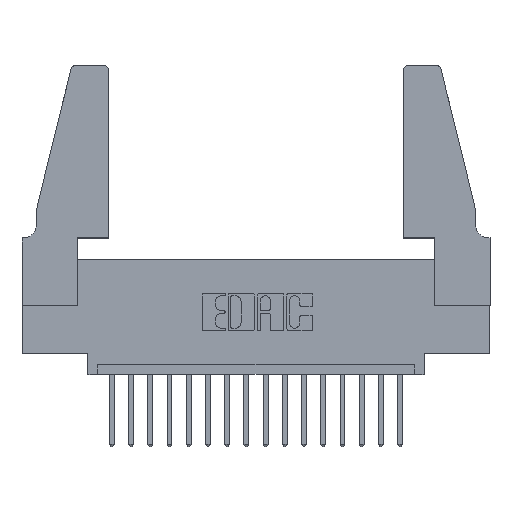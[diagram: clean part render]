
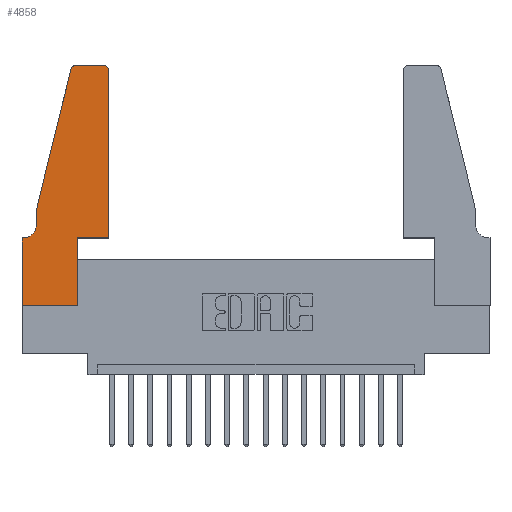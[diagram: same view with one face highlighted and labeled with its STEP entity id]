
A CAD part, top view. The second image highlights one B-rep face of the part: STEP entity #4858.
In plain terms, the highlighted planar face has unit normal (0, 0, 1).
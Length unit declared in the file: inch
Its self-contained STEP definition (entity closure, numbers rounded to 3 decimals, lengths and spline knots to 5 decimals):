
#25 = CARTESIAN_POINT ( 'NONE',  ( 0.4505, 0.35, 0.37 ) ) ;
#268 = EDGE_CURVE ( 'NONE', #8774, #3133, #7131, .T. ) ;
#560 = LINE ( 'NONE', #14806, #11050 ) ;
#875 = CARTESIAN_POINT ( 'NONE',  ( 0.2865, 0.35, 0.37 ) ) ;
#986 = CARTESIAN_POINT ( 'NONE',  ( 0.2865, 0.35, 0.37 ) ) ;
#1124 = EDGE_CURVE ( 'NONE', #5325, #8774, #1185, .T. ) ;
#1141 = ORIENTED_EDGE ( 'NONE', *, *, #7953, .T. ) ;
#1185 = LINE ( 'NONE', #986, #7198 ) ;
#1199 = DIRECTION ( 'NONE',  ( 1., 0., 0. ) ) ;
#1319 = VERTEX_POINT ( 'NONE', #6841 ) ;
#1401 = CARTESIAN_POINT ( 'NONE',  ( 0.0055, 0.42, 0.37 ) ) ;
#1741 = DIRECTION ( 'NONE',  ( -1., 0., 0. ) ) ;
#2296 = VECTOR ( 'NONE', #4685, 39.37008 ) ;
#2375 = DIRECTION ( 'NONE',  ( -1., 0., 0. ) ) ;
#2564 = ORIENTED_EDGE ( 'NONE', *, *, #8250, .T. ) ;
#2803 = DIRECTION ( 'NONE',  ( 1., 0., 0. ) ) ;
#3133 = VERTEX_POINT ( 'NONE', #7202 ) ;
#3313 = VECTOR ( 'NONE', #2375, 39.37008 ) ;
#3562 = VERTEX_POINT ( 'NONE', #12331 ) ;
#3579 = VERTEX_POINT ( 'NONE', #12566 ) ;
#3792 = CARTESIAN_POINT ( 'NONE',  ( 0., 0.35, 0.37 ) ) ;
#3866 = DIRECTION ( 'NONE',  ( 0., 1., 0. ) ) ;
#4262 = VERTEX_POINT ( 'NONE', #10989 ) ;
#4298 = CARTESIAN_POINT ( 'NONE',  ( 0.0755, 0.42, 0.37 ) ) ;
#4301 = AXIS2_PLACEMENT_3D ( 'NONE', #6587, #17739, #1199 ) ;
#4428 = LINE ( 'NONE', #6195, #2296 ) ;
#4685 = DIRECTION ( 'NONE',  ( -0.239, -0.971, 0. ) ) ;
#4858 = ADVANCED_FACE ( 'NONE', ( #16996 ), #9367, .T. ) ;
#4866 = LINE ( 'NONE', #14162, #9160 ) ;
#5049 = LINE ( 'NONE', #15166, #8493 ) ;
#5102 = CARTESIAN_POINT ( 'NONE',  ( 0.2865, 0., 0.37 ) ) ;
#5199 = CIRCLE ( 'NONE', #6097, 0.03 ) ;
#5325 = VERTEX_POINT ( 'NONE', #5102 ) ;
#5746 = DIRECTION ( 'NONE',  ( 1., 0., 0. ) ) ;
#6097 = AXIS2_PLACEMENT_3D ( 'NONE', #13949, #13835, #5746 ) ;
#6195 = CARTESIAN_POINT ( 'NONE',  ( 0.0755, 0.5, 0.37 ) ) ;
#6388 = DIRECTION ( 'NONE',  ( 0., 1., 0. ) ) ;
#6435 = ORIENTED_EDGE ( 'NONE', *, *, #17171, .T. ) ;
#6513 = ORIENTED_EDGE ( 'NONE', *, *, #9025, .T. ) ;
#6587 = CARTESIAN_POINT ( 'NONE',  ( 0.4205, 1.22, 0.37 ) ) ;
#6841 = CARTESIAN_POINT ( 'NONE',  ( 0., 0., 0.37 ) ) ;
#6978 = LINE ( 'NONE', #10558, #3313 ) ;
#7131 = LINE ( 'NONE', #25, #10958 ) ;
#7132 = DIRECTION ( 'NONE',  ( 0., -1., 0. ) ) ;
#7198 = VECTOR ( 'NONE', #6388, 39.37008 ) ;
#7202 = CARTESIAN_POINT ( 'NONE',  ( 0.4505, 0.35, 0.37 ) ) ;
#7537 = ORIENTED_EDGE ( 'NONE', *, *, #10752, .T. ) ;
#7682 = CARTESIAN_POINT ( 'NONE',  ( 0.0055, 0.35, 0.37 ) ) ;
#7765 = LINE ( 'NONE', #8574, #16847 ) ;
#7808 = EDGE_LOOP ( 'NONE', ( #1141, #11427, #2564, #12625, #10492, #16204, #7537, #12334, #12401, #11277, #6513, #6435 ) ) ;
#7953 = EDGE_CURVE ( 'NONE', #15549, #12107, #4866, .T. ) ;
#8250 = EDGE_CURVE ( 'NONE', #3579, #4262, #4428, .T. ) ;
#8289 = CARTESIAN_POINT ( 'NONE',  ( 0.4505, 1.22, 0.37 ) ) ;
#8493 = VECTOR ( 'NONE', #10809, 39.37008 ) ;
#8574 = CARTESIAN_POINT ( 'NONE',  ( 0., 0., 0.37 ) ) ;
#8774 = VERTEX_POINT ( 'NONE', #875 ) ;
#9025 = EDGE_CURVE ( 'NONE', #3133, #11017, #560, .T. ) ;
#9160 = VECTOR ( 'NONE', #1741, 39.37008 ) ;
#9367 = PLANE ( 'NONE',  #10485 ) ;
#9583 = EDGE_CURVE ( 'NONE', #11639, #3562, #6978, .T. ) ;
#10456 = EDGE_CURVE ( 'NONE', #12107, #3579, #5199, .T. ) ;
#10485 = AXIS2_PLACEMENT_3D ( 'NONE', #3792, #16322, #14791 ) ;
#10492 = ORIENTED_EDGE ( 'NONE', *, *, #13800, .T. ) ;
#10558 = CARTESIAN_POINT ( 'NONE',  ( 0.0755, 0.35, 0.37 ) ) ;
#10690 = CARTESIAN_POINT ( 'NONE',  ( 0.284, 1.25, 0.37 ) ) ;
#10752 = EDGE_CURVE ( 'NONE', #3562, #1319, #7765, .T. ) ;
#10809 = DIRECTION ( 'NONE',  ( 1., 0., 0. ) ) ;
#10958 = VECTOR ( 'NONE', #2803, 39.37008 ) ;
#10973 = DIRECTION ( 'NONE',  ( 0., 0., -1. ) ) ;
#10989 = CARTESIAN_POINT ( 'NONE',  ( 0.0755, 0.5, 0.37 ) ) ;
#11017 = VERTEX_POINT ( 'NONE', #8289 ) ;
#11050 = VECTOR ( 'NONE', #3866, 39.37008 ) ;
#11277 = ORIENTED_EDGE ( 'NONE', *, *, #268, .T. ) ;
#11427 = ORIENTED_EDGE ( 'NONE', *, *, #10456, .T. ) ;
#11463 = VERTEX_POINT ( 'NONE', #4298 ) ;
#11639 = VERTEX_POINT ( 'NONE', #7682 ) ;
#12107 = VERTEX_POINT ( 'NONE', #10690 ) ;
#12331 = CARTESIAN_POINT ( 'NONE',  ( 0., 0.35, 0.37 ) ) ;
#12334 = ORIENTED_EDGE ( 'NONE', *, *, #16058, .T. ) ;
#12363 = DIRECTION ( 'NONE',  ( -1., 0., 0. ) ) ;
#12401 = ORIENTED_EDGE ( 'NONE', *, *, #1124, .T. ) ;
#12566 = CARTESIAN_POINT ( 'NONE',  ( 0.25487, 1.22718, 0.37 ) ) ;
#12584 = DIRECTION ( 'NONE',  ( 0., -1., 0. ) ) ;
#12625 = ORIENTED_EDGE ( 'NONE', *, *, #15482, .T. ) ;
#12964 = CIRCLE ( 'NONE', #4301, 0.03 ) ;
#13785 = CARTESIAN_POINT ( 'NONE',  ( 0.4205, 1.25, 0.37 ) ) ;
#13800 = EDGE_CURVE ( 'NONE', #11463, #11639, #17616, .T. ) ;
#13835 = DIRECTION ( 'NONE',  ( 0., 0., 1. ) ) ;
#13846 = CARTESIAN_POINT ( 'NONE',  ( 0.0755, 0.5, 0.37 ) ) ;
#13949 = CARTESIAN_POINT ( 'NONE',  ( 0.284, 1.22, 0.37 ) ) ;
#14162 = CARTESIAN_POINT ( 'NONE',  ( 0.2605, 1.25, 0.37 ) ) ;
#14188 = AXIS2_PLACEMENT_3D ( 'NONE', #1401, #10973, #12363 ) ;
#14791 = DIRECTION ( 'NONE',  ( 1., 0., 0. ) ) ;
#14806 = CARTESIAN_POINT ( 'NONE',  ( 0.4505, 0.35, 0.37 ) ) ;
#14979 = LINE ( 'NONE', #13846, #17587 ) ;
#15166 = CARTESIAN_POINT ( 'NONE',  ( 0., 0., 0.37 ) ) ;
#15482 = EDGE_CURVE ( 'NONE', #4262, #11463, #14979, .T. ) ;
#15549 = VERTEX_POINT ( 'NONE', #13785 ) ;
#16058 = EDGE_CURVE ( 'NONE', #1319, #5325, #5049, .T. ) ;
#16204 = ORIENTED_EDGE ( 'NONE', *, *, #9583, .T. ) ;
#16322 = DIRECTION ( 'NONE',  ( 0., 0., 1. ) ) ;
#16847 = VECTOR ( 'NONE', #12584, 39.37008 ) ;
#16996 = FACE_OUTER_BOUND ( 'NONE', #7808, .T. ) ;
#17171 = EDGE_CURVE ( 'NONE', #11017, #15549, #12964, .T. ) ;
#17587 = VECTOR ( 'NONE', #7132, 39.37008 ) ;
#17616 = CIRCLE ( 'NONE', #14188, 0.07 ) ;
#17739 = DIRECTION ( 'NONE',  ( 0., 0., 1. ) ) ;
